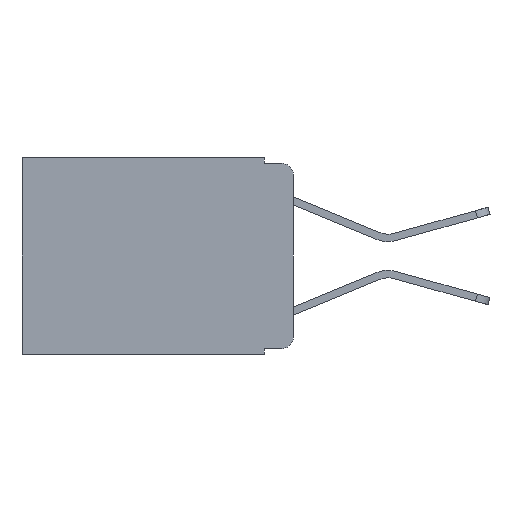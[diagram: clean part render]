
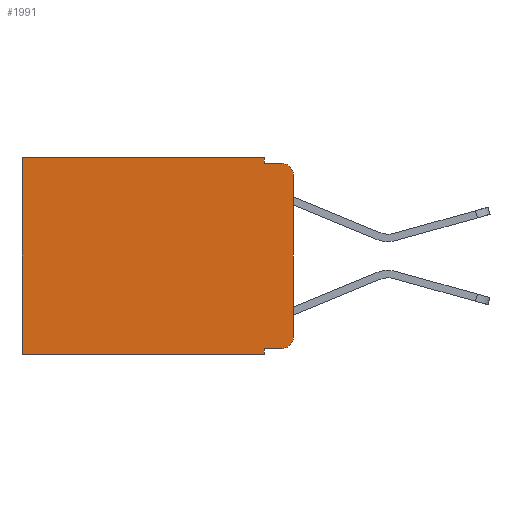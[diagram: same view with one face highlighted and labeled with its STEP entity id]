
A CAD part, left-side view. The second image highlights one B-rep face of the part: STEP entity #1991.
In plain terms, the highlighted planar face has unit normal (-1, 0, 0).
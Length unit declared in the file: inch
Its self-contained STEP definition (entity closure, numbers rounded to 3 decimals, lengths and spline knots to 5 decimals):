
#292 = CARTESIAN_POINT ( 'NONE',  ( 0.298, 0.02, -0.313 ) ) ;
#452 = ORIENTED_EDGE ( 'NONE', *, *, #3731, .F. ) ;
#568 = AXIS2_PLACEMENT_3D ( 'NONE', #8546, #10405, #3704 ) ;
#670 = DIRECTION ( 'NONE',  ( 0., -1., 0. ) ) ;
#772 = EDGE_CURVE ( 'NONE', #2364, #7026, #8075, .T. ) ;
#855 = CARTESIAN_POINT ( 'NONE',  ( 0.298, 0.051, -0.333 ) ) ;
#928 = CARTESIAN_POINT ( 'NONE',  ( 0.298, 0.051, 0. ) ) ;
#1092 = CARTESIAN_POINT ( 'NONE',  ( 0.298, 0.02, -0.333 ) ) ;
#1097 = VECTOR ( 'NONE', #6493, 39.37008 ) ;
#1317 = DIRECTION ( 'NONE',  ( 0., 0., -1. ) ) ;
#1648 = EDGE_CURVE ( 'NONE', #4304, #7762, #2736, .T. ) ;
#1781 = EDGE_CURVE ( 'NONE', #6711, #7026, #10860, .T. ) ;
#1882 = CARTESIAN_POINT ( 'NONE',  ( 0.298, 0.051, -0.343 ) ) ;
#1989 = EDGE_CURVE ( 'NONE', #2560, #2364, #2164, .T. ) ;
#1991 = ADVANCED_FACE ( 'NONE', ( #4154 ), #10179, .F. ) ;
#2024 = ORIENTED_EDGE ( 'NONE', *, *, #7538, .F. ) ;
#2147 = ORIENTED_EDGE ( 'NONE', *, *, #1781, .F. ) ;
#2164 = LINE ( 'NONE', #8820, #8534 ) ;
#2316 = VECTOR ( 'NONE', #9431, 39.37008 ) ;
#2364 = VERTEX_POINT ( 'NONE', #1092 ) ;
#2528 = CARTESIAN_POINT ( 'NONE',  ( 0.298, 0., -0.313 ) ) ;
#2560 = VERTEX_POINT ( 'NONE', #855 ) ;
#2565 = VECTOR ( 'NONE', #1317, 39.37008 ) ;
#2736 = LINE ( 'NONE', #6341, #8791 ) ;
#2889 = LINE ( 'NONE', #8586, #4861 ) ;
#3005 = ORIENTED_EDGE ( 'NONE', *, *, #4862, .T. ) ;
#3567 = ORIENTED_EDGE ( 'NONE', *, *, #772, .T. ) ;
#3632 = CARTESIAN_POINT ( 'NONE',  ( 0.298, 0.051, 0. ) ) ;
#3691 = LINE ( 'NONE', #928, #1097 ) ;
#3704 = DIRECTION ( 'NONE',  ( 0., 0., -1. ) ) ;
#3731 = EDGE_CURVE ( 'NONE', #2560, #6559, #6974, .T. ) ;
#4067 = ORIENTED_EDGE ( 'NONE', *, *, #8683, .F. ) ;
#4109 = DIRECTION ( 'NONE',  ( 0., 0., -1. ) ) ;
#4137 = DIRECTION ( 'NONE',  ( 0., 1., 0. ) ) ;
#4154 = FACE_OUTER_BOUND ( 'NONE', #9802, .T. ) ;
#4304 = VERTEX_POINT ( 'NONE', #4677 ) ;
#4329 = CARTESIAN_POINT ( 'NONE',  ( 0.298, 0.02, -0.01 ) ) ;
#4442 = CARTESIAN_POINT ( 'NONE',  ( 0.298, 0.051, -0.01 ) ) ;
#4677 = CARTESIAN_POINT ( 'NONE',  ( 0.298, 0.051, 0. ) ) ;
#4861 = VECTOR ( 'NONE', #7646, 39.37008 ) ;
#4862 = EDGE_CURVE ( 'NONE', #7762, #8953, #5565, .T. ) ;
#5165 = CARTESIAN_POINT ( 'NONE',  ( 0.298, 0.473, 0. ) ) ;
#5326 = CARTESIAN_POINT ( 'NONE',  ( 0.298, 0.051, -0.01 ) ) ;
#5430 = CARTESIAN_POINT ( 'NONE',  ( 0.298, 0., -0.03 ) ) ;
#5565 = LINE ( 'NONE', #5165, #5816 ) ;
#5816 = VECTOR ( 'NONE', #4109, 39.37008 ) ;
#5971 = EDGE_CURVE ( 'NONE', #4304, #6694, #3691, .T. ) ;
#6020 = CARTESIAN_POINT ( 'NONE',  ( 0.298, 0.473, -0.343 ) ) ;
#6341 = CARTESIAN_POINT ( 'NONE',  ( 0.298, 0., 0. ) ) ;
#6493 = DIRECTION ( 'NONE',  ( 0., 0., -1. ) ) ;
#6559 = VERTEX_POINT ( 'NONE', #1882 ) ;
#6694 = VERTEX_POINT ( 'NONE', #5326 ) ;
#6711 = VERTEX_POINT ( 'NONE', #5430 ) ;
#6974 = LINE ( 'NONE', #3632, #2565 ) ;
#7026 = VERTEX_POINT ( 'NONE', #2528 ) ;
#7538 = EDGE_CURVE ( 'NONE', #6559, #8953, #2889, .T. ) ;
#7646 = DIRECTION ( 'NONE',  ( 0., 1., 0. ) ) ;
#7762 = VERTEX_POINT ( 'NONE', #10156 ) ;
#8050 = ORIENTED_EDGE ( 'NONE', *, *, #9817, .T. ) ;
#8075 = CIRCLE ( 'NONE', #8703, 0.02 ) ;
#8122 = CARTESIAN_POINT ( 'NONE',  ( 0.298, 0., 0. ) ) ;
#8160 = ORIENTED_EDGE ( 'NONE', *, *, #5971, .F. ) ;
#8516 = DIRECTION ( 'NONE',  ( 0., -1., 0. ) ) ;
#8534 = VECTOR ( 'NONE', #670, 39.37008 ) ;
#8546 = CARTESIAN_POINT ( 'NONE',  ( 0.298, 0.02, -0.03 ) ) ;
#8586 = CARTESIAN_POINT ( 'NONE',  ( 0.298, 0., -0.343 ) ) ;
#8683 = EDGE_CURVE ( 'NONE', #6694, #9403, #8778, .T. ) ;
#8703 = AXIS2_PLACEMENT_3D ( 'NONE', #292, #9310, #9321 ) ;
#8778 = LINE ( 'NONE', #4442, #10499 ) ;
#8791 = VECTOR ( 'NONE', #4137, 39.37008 ) ;
#8820 = CARTESIAN_POINT ( 'NONE',  ( 0.298, 0.051, -0.333 ) ) ;
#8953 = VERTEX_POINT ( 'NONE', #6020 ) ;
#8979 = AXIS2_PLACEMENT_3D ( 'NONE', #8122, #10916, #10901 ) ;
#9303 = ORIENTED_EDGE ( 'NONE', *, *, #1648, .T. ) ;
#9310 = DIRECTION ( 'NONE',  ( -1., 0., 0. ) ) ;
#9321 = DIRECTION ( 'NONE',  ( 0., 0., -1. ) ) ;
#9403 = VERTEX_POINT ( 'NONE', #4329 ) ;
#9431 = DIRECTION ( 'NONE',  ( 0., 0., -1. ) ) ;
#9760 = CARTESIAN_POINT ( 'NONE',  ( 0.298, 0., 0. ) ) ;
#9802 = EDGE_LOOP ( 'NONE', ( #2147, #8050, #4067, #8160, #9303, #3005, #2024, #452, #10404, #3567 ) ) ;
#9817 = EDGE_CURVE ( 'NONE', #6711, #9403, #10594, .T. ) ;
#10156 = CARTESIAN_POINT ( 'NONE',  ( 0.298, 0.473, 0. ) ) ;
#10179 = PLANE ( 'NONE',  #8979 ) ;
#10404 = ORIENTED_EDGE ( 'NONE', *, *, #1989, .T. ) ;
#10405 = DIRECTION ( 'NONE',  ( -1., 0., 0. ) ) ;
#10499 = VECTOR ( 'NONE', #8516, 39.37008 ) ;
#10594 = CIRCLE ( 'NONE', #568, 0.02 ) ;
#10860 = LINE ( 'NONE', #9760, #2316 ) ;
#10901 = DIRECTION ( 'NONE',  ( 0., 0., -1. ) ) ;
#10916 = DIRECTION ( 'NONE',  ( 1., 0., 0. ) ) ;
